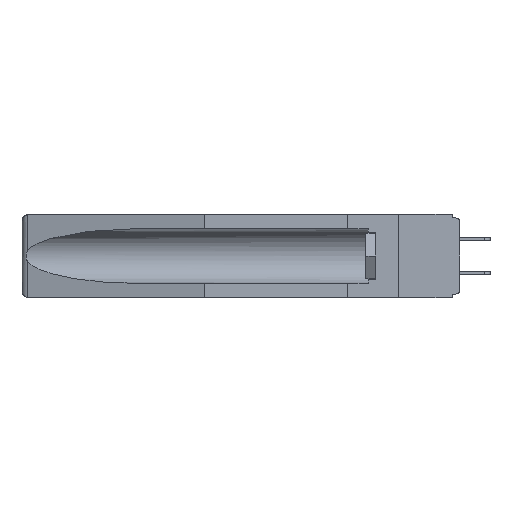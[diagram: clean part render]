
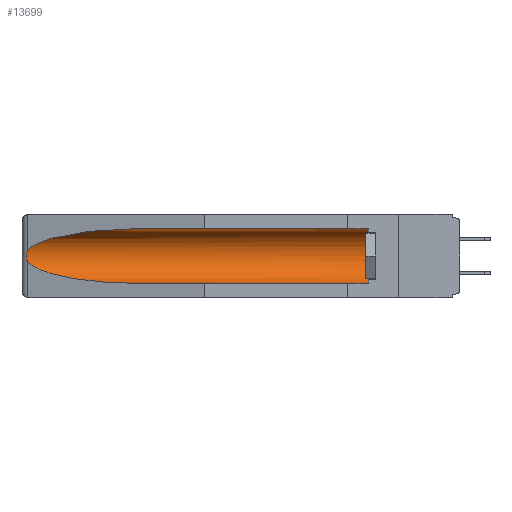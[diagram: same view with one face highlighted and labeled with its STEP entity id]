
A CAD part, left-side view. The second image highlights one B-rep face of the part: STEP entity #13699.
In plain terms, the highlighted cylindrical face has radius 2.857 mm (diameter 5.715 mm), a partial arc.
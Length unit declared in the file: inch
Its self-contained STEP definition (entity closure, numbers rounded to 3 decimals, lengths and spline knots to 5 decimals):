
#143 = CYLINDRICAL_SURFACE ( 'NONE', #16083, 0.1125 ) ;
#453 = CARTESIAN_POINT ( 'NONE',  ( 0.26537, 1.52718, -0.19328 ) ) ;
#489 = VERTEX_POINT ( 'NONE', #13454 ) ;
#498 = CARTESIAN_POINT ( 'NONE',  ( 0.155, 1.07973, -0.284 ) ) ;
#755 = CARTESIAN_POINT ( 'NONE',  ( 0.26654, 1.53092, -0.15636 ) ) ;
#780 = ORIENTED_EDGE ( 'NONE', *, *, #1691, .T. ) ;
#930 = CARTESIAN_POINT ( 'NONE',  ( 0.2673, 1.5327, -0.16383 ) ) ;
#1103 = DIRECTION ( 'NONE',  ( 0., 1., 0. ) ) ;
#1409 = VERTEX_POINT ( 'NONE', #498 ) ;
#1503 = CARTESIAN_POINT ( 'NONE',  ( 0.155, -0.30754, -0.1715 ) ) ;
#1691 = EDGE_CURVE ( 'NONE', #13134, #489, #4903, .T. ) ;
#2125 = CARTESIAN_POINT ( 'NONE',  ( 0.26655, 1.53094, -0.18657 ) ) ;
#2347 = ORIENTED_EDGE ( 'NONE', *, *, #11697, .T. ) ;
#2352 = LINE ( 'NONE', #6608, #16748 ) ;
#3376 = ORIENTED_EDGE ( 'NONE', *, *, #14429, .T. ) ;
#3447 = DIRECTION ( 'NONE',  ( 0., 0., 1. ) ) ;
#4362 = VECTOR ( 'NONE', #5780, 39.37008 ) ;
#4433 = CARTESIAN_POINT ( 'NONE',  ( 0.21114, 1.30732, -0.059 ) ) ;
#4617 = CARTESIAN_POINT ( 'NONE',  ( 0.25451, 1.48313, -0.09465 ) ) ;
#4903 = CIRCLE ( 'NONE', #5274, 0.1125 ) ;
#5274 = AXIS2_PLACEMENT_3D ( 'NONE', #11827, #10647, #3447 ) ;
#5780 = DIRECTION ( 'NONE',  ( 0., 1., 0. ) ) ;
#5879 = CARTESIAN_POINT ( 'NONE',  ( 0.155, 1.07973, -0.059 ) ) ;
#6608 = CARTESIAN_POINT ( 'NONE',  ( 0.155, -0.30754, -0.059 ) ) ;
#7012 = ORIENTED_EDGE ( 'NONE', *, *, #16685, .T. ) ;
#7417 = CARTESIAN_POINT ( 'NONE',  ( 0.155, 1.07973, -0.284 ) ) ;
#7429 = VERTEX_POINT ( 'NONE', #12249 ) ;
#7739 = CARTESIAN_POINT ( 'NONE',  ( 0.2673, 1.53269, -0.17917 ) ) ;
#7798 = CARTESIAN_POINT ( 'NONE',  ( 0.26597, 1.5296, -0.19026 ) ) ;
#9083 = CARTESIAN_POINT ( 'NONE',  ( 0.26597, 1.52961, -0.15275 ) ) ;
#9133 =( BOUNDED_CURVE ( )  B_SPLINE_CURVE ( 3, ( #5879, #4433, #4617, #17075 ),
 .UNSPECIFIED., .F., .F. ) 
 B_SPLINE_CURVE_WITH_KNOTS ( ( 4, 4 ),
 ( 4.71239, 6.08839 ),
 .UNSPECIFIED. ) 
 CURVE ( )  GEOMETRIC_REPRESENTATION_ITEM ( )  RATIONAL_B_SPLINE_CURVE ( ( 1., 0.848, 0.848, 1. ) ) 
 REPRESENTATION_ITEM ( '' )  );
#10357 = FACE_OUTER_BOUND ( 'NONE', #16037, .T. ) ;
#10647 = DIRECTION ( 'NONE',  ( 0., -1., 0. ) ) ;
#11281 =( BOUNDED_CURVE ( )  B_SPLINE_CURVE ( 3, ( #453, #14300, #17107, #7417 ),
 .UNSPECIFIED., .F., .F. ) 
 B_SPLINE_CURVE_WITH_KNOTS ( ( 4, 4 ),
 ( 0.1948, 1.5708 ),
 .UNSPECIFIED. ) 
 CURVE ( )  GEOMETRIC_REPRESENTATION_ITEM ( )  RATIONAL_B_SPLINE_CURVE ( ( 1., 0.848, 0.848, 1. ) ) 
 REPRESENTATION_ITEM ( '' )  );
#11391 = EDGE_CURVE ( 'NONE', #489, #11552, #2352, .T. ) ;
#11552 = VERTEX_POINT ( 'NONE', #17910 ) ;
#11697 = EDGE_CURVE ( 'NONE', #14302, #1409, #11281, .T. ) ;
#11821 = LINE ( 'NONE', #16841, #4362 ) ;
#11827 = CARTESIAN_POINT ( 'NONE',  ( 0.155, 0.126, -0.1715 ) ) ;
#12249 = CARTESIAN_POINT ( 'NONE',  ( 0.26537, 1.52718, -0.14972 ) ) ;
#12735 = ORIENTED_EDGE ( 'NONE', *, *, #15576, .F. ) ;
#13134 = VERTEX_POINT ( 'NONE', #13874 ) ;
#13454 = CARTESIAN_POINT ( 'NONE',  ( 0.155, 0.126, -0.059 ) ) ;
#13458 = CARTESIAN_POINT ( 'NONE',  ( 0.2675, 1.53308, -0.16763 ) ) ;
#13699 = ADVANCED_FACE ( 'NONE', ( #10357 ), #143, .F. ) ;
#13874 = CARTESIAN_POINT ( 'NONE',  ( 0.155, 0.126, -0.284 ) ) ;
#14284 = B_SPLINE_CURVE_WITH_KNOTS ( 'NONE', 3,
 ( #17612, #9083, #755, #930, #13458, #14774, #7739, #2125, #7798, #14611 ),
 .UNSPECIFIED., .F., .F.,
 ( 4, 2, 2, 2, 4 ),
 ( 0., 0.00029, 0.00058, 0.00087, 0.00117 ),
 .UNSPECIFIED. ) ;
#14300 = CARTESIAN_POINT ( 'NONE',  ( 0.25451, 1.48313, -0.24835 ) ) ;
#14302 = VERTEX_POINT ( 'NONE', #16817 ) ;
#14385 = ORIENTED_EDGE ( 'NONE', *, *, #11391, .T. ) ;
#14429 = EDGE_CURVE ( 'NONE', #11552, #7429, #9133, .T. ) ;
#14611 = CARTESIAN_POINT ( 'NONE',  ( 0.26537, 1.52718, -0.19328 ) ) ;
#14774 = CARTESIAN_POINT ( 'NONE',  ( 0.2675, 1.53308, -0.17534 ) ) ;
#15576 = EDGE_CURVE ( 'NONE', #13134, #1409, #11821, .T. ) ;
#16037 = EDGE_LOOP ( 'NONE', ( #3376, #7012, #2347, #12735, #780, #14385 ) ) ;
#16083 = AXIS2_PLACEMENT_3D ( 'NONE', #1503, #16584, #16784 ) ;
#16584 = DIRECTION ( 'NONE',  ( 0., 1., 0. ) ) ;
#16685 = EDGE_CURVE ( 'NONE', #7429, #14302, #14284, .T. ) ;
#16748 = VECTOR ( 'NONE', #1103, 39.37008 ) ;
#16784 = DIRECTION ( 'NONE',  ( 0., 0., 1. ) ) ;
#16817 = CARTESIAN_POINT ( 'NONE',  ( 0.26537, 1.52718, -0.19328 ) ) ;
#16841 = CARTESIAN_POINT ( 'NONE',  ( 0.155, -0.30754, -0.284 ) ) ;
#17075 = CARTESIAN_POINT ( 'NONE',  ( 0.26537, 1.52718, -0.14972 ) ) ;
#17107 = CARTESIAN_POINT ( 'NONE',  ( 0.21114, 1.30732, -0.284 ) ) ;
#17612 = CARTESIAN_POINT ( 'NONE',  ( 0.26537, 1.52718, -0.14972 ) ) ;
#17910 = CARTESIAN_POINT ( 'NONE',  ( 0.155, 1.07973, -0.059 ) ) ;
